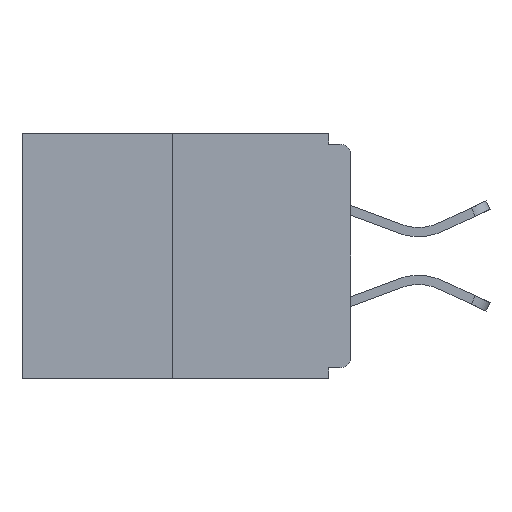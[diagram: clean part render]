
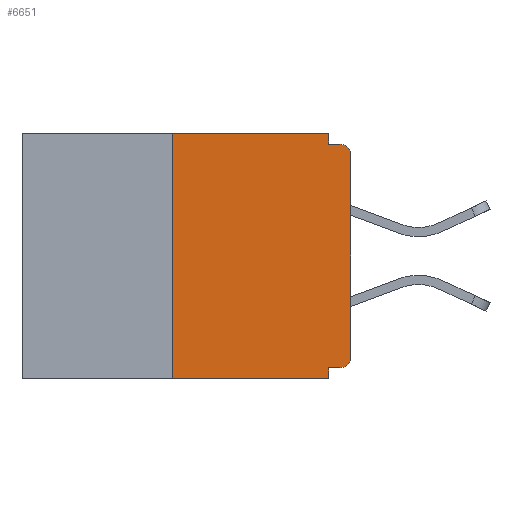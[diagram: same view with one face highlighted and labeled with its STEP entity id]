
A CAD part, left-side view. The second image highlights one B-rep face of the part: STEP entity #6651.
In plain terms, the highlighted planar face has unit normal (-1, 0, 0).
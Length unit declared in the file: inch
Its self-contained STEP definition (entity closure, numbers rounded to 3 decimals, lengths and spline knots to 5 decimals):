
#65 = DIRECTION ( 'NONE',  ( 0., -1., 0. ) ) ;
#79 = DIRECTION ( 'NONE',  ( 0., 0., -1. ) ) ;
#128 = CIRCLE ( 'NONE', #11876, 0.015 ) ;
#210 = VERTEX_POINT ( 'NONE', #13676 ) ;
#213 = DIRECTION ( 'NONE',  ( -1., 0., 0. ) ) ;
#855 = CARTESIAN_POINT ( 'NONE',  ( 0., 0.46, 0. ) ) ;
#1349 = LINE ( 'NONE', #6999, #19672 ) ;
#1719 = CARTESIAN_POINT ( 'NONE',  ( 0., 0.031, -0.343 ) ) ;
#1870 = CARTESIAN_POINT ( 'NONE',  ( 0., 0.031, -0.015 ) ) ;
#2713 = VERTEX_POINT ( 'NONE', #10285 ) ;
#3565 = CARTESIAN_POINT ( 'NONE',  ( 0., 0.031, -0.328 ) ) ;
#5007 = CIRCLE ( 'NONE', #15927, 0.015 ) ;
#5162 = ORIENTED_EDGE ( 'NONE', *, *, #24696, .F. ) ;
#5629 = DIRECTION ( 'NONE',  ( 0., 0., 1. ) ) ;
#5783 = DIRECTION ( 'NONE',  ( 0., 0., -1. ) ) ;
#5978 = ORIENTED_EDGE ( 'NONE', *, *, #18400, .T. ) ;
#6072 = DIRECTION ( 'NONE',  ( 0., 1., 0. ) ) ;
#6278 = EDGE_CURVE ( 'NONE', #210, #8530, #128, .T. ) ;
#6455 = LINE ( 'NONE', #10657, #21915 ) ;
#6651 = ADVANCED_FACE ( 'NONE', ( #20837 ), #23321, .F. ) ;
#6999 = CARTESIAN_POINT ( 'NONE',  ( 0., 0.46, -0.343 ) ) ;
#7777 = CARTESIAN_POINT ( 'NONE',  ( 0., 0., -0.328 ) ) ;
#7815 = ORIENTED_EDGE ( 'NONE', *, *, #14753, .T. ) ;
#8064 = DIRECTION ( 'NONE',  ( 0., 0., -1. ) ) ;
#8352 = CARTESIAN_POINT ( 'NONE',  ( 0., 0.015, -0.015 ) ) ;
#8530 = VERTEX_POINT ( 'NONE', #24416 ) ;
#8613 = VECTOR ( 'NONE', #11745, 39.37008 ) ;
#9039 = ORIENTED_EDGE ( 'NONE', *, *, #6278, .T. ) ;
#9641 = CARTESIAN_POINT ( 'NONE',  ( 0., 0., 0. ) ) ;
#10285 = CARTESIAN_POINT ( 'NONE',  ( 0., 0.031, -0.343 ) ) ;
#10386 = EDGE_CURVE ( 'NONE', #13968, #12484, #14226, .T. ) ;
#10531 = VERTEX_POINT ( 'NONE', #14888 ) ;
#10657 = CARTESIAN_POINT ( 'NONE',  ( 0., 0.031, 0. ) ) ;
#10678 = VERTEX_POINT ( 'NONE', #3565 ) ;
#11332 = DIRECTION ( 'NONE',  ( 0., 0., -1. ) ) ;
#11716 = LINE ( 'NONE', #7777, #18667 ) ;
#11745 = DIRECTION ( 'NONE',  ( 0., 0., 1. ) ) ;
#11876 = AXIS2_PLACEMENT_3D ( 'NONE', #14013, #15718, #79 ) ;
#11967 = EDGE_LOOP ( 'NONE', ( #23861, #21797, #22033, #21541, #21166, #9039, #5978, #7815, #23977, #5162 ) ) ;
#12370 = EDGE_CURVE ( 'NONE', #10531, #21478, #15617, .T. ) ;
#12405 = CARTESIAN_POINT ( 'NONE',  ( 0., 0.031, 0. ) ) ;
#12484 = VERTEX_POINT ( 'NONE', #8352 ) ;
#13518 = EDGE_CURVE ( 'NONE', #21478, #23073, #22017, .T. ) ;
#13676 = CARTESIAN_POINT ( 'NONE',  ( 0., 0.015, -0.328 ) ) ;
#13945 = EDGE_CURVE ( 'NONE', #210, #10678, #11716, .T. ) ;
#13968 = VERTEX_POINT ( 'NONE', #1870 ) ;
#14013 = CARTESIAN_POINT ( 'NONE',  ( 0., 0.015, -0.313 ) ) ;
#14226 = LINE ( 'NONE', #15925, #17415 ) ;
#14753 = EDGE_CURVE ( 'NONE', #23609, #12484, #5007, .T. ) ;
#14888 = CARTESIAN_POINT ( 'NONE',  ( 0., 0.25, -0.343 ) ) ;
#15027 = DIRECTION ( 'NONE',  ( 0., -1., 0. ) ) ;
#15264 = CARTESIAN_POINT ( 'NONE',  ( 0., 0., -0.03 ) ) ;
#15617 = LINE ( 'NONE', #23637, #16140 ) ;
#15718 = DIRECTION ( 'NONE',  ( -1., 0., 0. ) ) ;
#15902 = CARTESIAN_POINT ( 'NONE',  ( 0., 0.25, 0. ) ) ;
#15925 = CARTESIAN_POINT ( 'NONE',  ( 0., 0., -0.015 ) ) ;
#15927 = AXIS2_PLACEMENT_3D ( 'NONE', #18070, #213, #8064 ) ;
#16140 = VECTOR ( 'NONE', #5629, 39.37008 ) ;
#16591 = DIRECTION ( 'NONE',  ( 0., 0., -1. ) ) ;
#16890 = DIRECTION ( 'NONE',  ( 1., 0., 0. ) ) ;
#17415 = VECTOR ( 'NONE', #21852, 39.37008 ) ;
#18070 = CARTESIAN_POINT ( 'NONE',  ( 0., 0.015, -0.03 ) ) ;
#18400 = EDGE_CURVE ( 'NONE', #8530, #23609, #25295, .T. ) ;
#18667 = VECTOR ( 'NONE', #6072, 39.37008 ) ;
#19672 = VECTOR ( 'NONE', #15027, 39.37008 ) ;
#20167 = CARTESIAN_POINT ( 'NONE',  ( 0., 0.46, 0. ) ) ;
#20607 = EDGE_CURVE ( 'NONE', #10531, #2713, #1349, .T. ) ;
#20688 = VECTOR ( 'NONE', #5783, 39.37008 ) ;
#20837 = FACE_OUTER_BOUND ( 'NONE', #11967, .T. ) ;
#21166 = ORIENTED_EDGE ( 'NONE', *, *, #13945, .F. ) ;
#21478 = VERTEX_POINT ( 'NONE', #15902 ) ;
#21541 = ORIENTED_EDGE ( 'NONE', *, *, #25569, .F. ) ;
#21797 = ORIENTED_EDGE ( 'NONE', *, *, #12370, .F. ) ;
#21852 = DIRECTION ( 'NONE',  ( 0., -1., 0. ) ) ;
#21915 = VECTOR ( 'NONE', #16591, 39.37008 ) ;
#22017 = LINE ( 'NONE', #20167, #24995 ) ;
#22033 = ORIENTED_EDGE ( 'NONE', *, *, #20607, .T. ) ;
#22434 = AXIS2_PLACEMENT_3D ( 'NONE', #855, #16890, #11332 ) ;
#23073 = VERTEX_POINT ( 'NONE', #12405 ) ;
#23321 = PLANE ( 'NONE',  #22434 ) ;
#23609 = VERTEX_POINT ( 'NONE', #15264 ) ;
#23637 = CARTESIAN_POINT ( 'NONE',  ( 0., 0.25, 0. ) ) ;
#23674 = LINE ( 'NONE', #1719, #20688 ) ;
#23861 = ORIENTED_EDGE ( 'NONE', *, *, #13518, .F. ) ;
#23977 = ORIENTED_EDGE ( 'NONE', *, *, #10386, .F. ) ;
#24416 = CARTESIAN_POINT ( 'NONE',  ( 0., 0., -0.313 ) ) ;
#24696 = EDGE_CURVE ( 'NONE', #23073, #13968, #6455, .T. ) ;
#24995 = VECTOR ( 'NONE', #65, 39.37008 ) ;
#25295 = LINE ( 'NONE', #9641, #8613 ) ;
#25569 = EDGE_CURVE ( 'NONE', #10678, #2713, #23674, .T. ) ;
